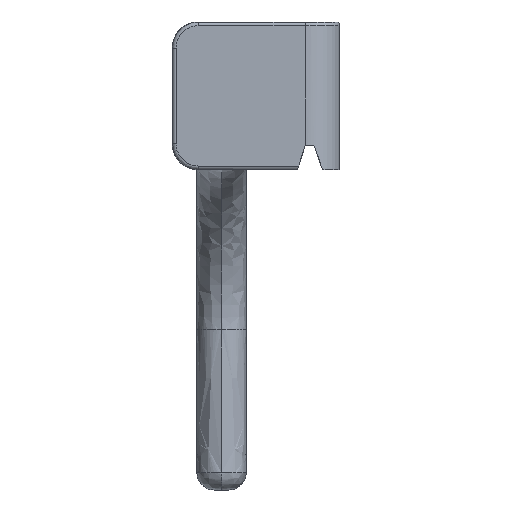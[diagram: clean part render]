
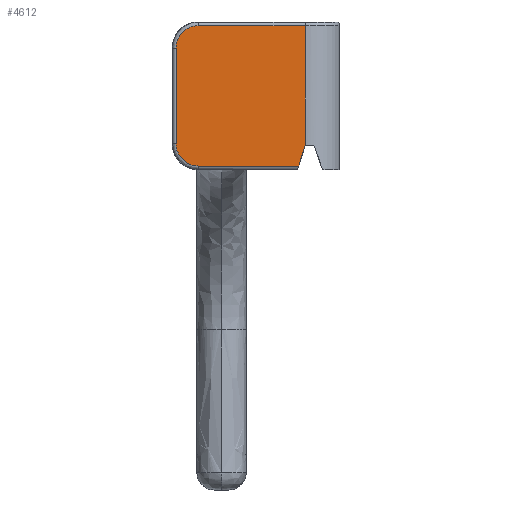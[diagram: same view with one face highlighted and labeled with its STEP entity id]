
A CAD part, front view. The second image highlights one B-rep face of the part: STEP entity #4612.
In plain terms, the highlighted planar face has unit normal (0, -1, 0).
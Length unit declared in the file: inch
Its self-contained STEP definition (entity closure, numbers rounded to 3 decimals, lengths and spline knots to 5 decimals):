
#20=PLANE('',#4950);
#330=FACE_OUTER_BOUND('',#638,.T.);
#638=EDGE_LOOP('',(#3064,#3065,#3066,#3067,#3068,#3069,#3070));
#939=B_SPLINE_CURVE_WITH_KNOTS('',3,(#5378,#5379,#5380,#5381,#5382,#5383),
 .UNSPECIFIED.,.F.,.F.,(4,1,1,4),(-0.71331,-0.40761,
-0.2038,0.),.UNSPECIFIED.);
#941=B_SPLINE_CURVE_WITH_KNOTS('',3,(#5429,#5430,#5431,#5432,#5433,#5434),
 .UNSPECIFIED.,.F.,.F.,(4,1,1,4),(-0.71331,-0.50951,
-0.3057,0.),.UNSPECIFIED.);
#1635=LINE('',#5343,#1679);
#1637=LINE('',#5394,#1681);
#1639=LINE('',#5445,#1683);
#1646=LINE('',#5490,#1690);
#1647=LINE('',#5497,#1691);
#1679=VECTOR('',#5064,0.3937);
#1681=VECTOR('',#5072,0.3937);
#1683=VECTOR('',#5080,0.3937);
#1690=VECTOR('',#5099,0.3937);
#1691=VECTOR('',#5108,0.3937);
#1769=VERTEX_POINT('',#5335);
#1771=VERTEX_POINT('',#5341);
#1773=VERTEX_POINT('',#5376);
#1775=VERTEX_POINT('',#5392);
#1777=VERTEX_POINT('',#5427);
#1779=VERTEX_POINT('',#5443);
#1788=VERTEX_POINT('',#5489);
#2237=EDGE_CURVE('',#1771,#1769,#1635,.T.);
#2240=EDGE_CURVE('',#1773,#1771,#939,.T.);
#2243=EDGE_CURVE('',#1775,#1773,#1637,.T.);
#2246=EDGE_CURVE('',#1777,#1775,#941,.T.);
#2249=EDGE_CURVE('',#1779,#1777,#1639,.T.);
#2261=EDGE_CURVE('',#1769,#1788,#1646,.T.);
#2265=EDGE_CURVE('',#1779,#1788,#1647,.T.);
#3064=ORIENTED_EDGE('',*,*,#2237,.F.);
#3065=ORIENTED_EDGE('',*,*,#2240,.F.);
#3066=ORIENTED_EDGE('',*,*,#2243,.F.);
#3067=ORIENTED_EDGE('',*,*,#2246,.F.);
#3068=ORIENTED_EDGE('',*,*,#2249,.F.);
#3069=ORIENTED_EDGE('',*,*,#2265,.T.);
#3070=ORIENTED_EDGE('',*,*,#2261,.F.);
#4612=ADVANCED_FACE('',(#330),#20,.T.);
#4950=AXIS2_PLACEMENT_3D('',#5496,#5106,#5107);
#5064=DIRECTION('',(1.,0.,0.));
#5072=DIRECTION('',(0.,0.,1.));
#5080=DIRECTION('',(-1.,0.,0.));
#5099=DIRECTION('',(0.,0.,-1.));
#5106=DIRECTION('center_axis',(0.,-1.,0.));
#5107=DIRECTION('ref_axis',(0.,0.,
-1.));
#5108=DIRECTION('',(0.3,0.,0.954));
#5335=CARTESIAN_POINT('',(0.6717,3.13929,-1.06923));
#5341=CARTESIAN_POINT('',(-0.18251,3.13929,-1.06923));
#5343=CARTESIAN_POINT('',(-0.19445,3.13929,-1.06923));
#5376=CARTESIAN_POINT('',(-0.3613,3.13929,-1.24802));
#5378=CARTESIAN_POINT('Ctrl Pts',(-0.3613,3.13929,-1.24802));
#5379=CARTESIAN_POINT('Ctrl Pts',(-0.3613,3.13929,-1.2079));
#5380=CARTESIAN_POINT('Ctrl Pts',(-0.33784,3.13929,-1.14128));
#5381=CARTESIAN_POINT('Ctrl Pts',(-0.26264,3.13929,-1.08147));
#5382=CARTESIAN_POINT('Ctrl Pts',(-0.20925,3.13929,-1.06923));
#5383=CARTESIAN_POINT('Ctrl Pts',(-0.18251,3.13929,-1.06923));
#5392=CARTESIAN_POINT('',(-0.3613,3.13929,-2.01154));
#5394=CARTESIAN_POINT('',(-0.3613,3.13929,-1.97427));
#5427=CARTESIAN_POINT('',(-0.18251,3.13929,-2.19033));
#5429=CARTESIAN_POINT('Ctrl Pts',(-0.18251,3.13929,-2.19033));
#5430=CARTESIAN_POINT('Ctrl Pts',(-0.20925,3.13929,-2.19033));
#5431=CARTESIAN_POINT('Ctrl Pts',(-0.26264,3.13929,-2.17809));
#5432=CARTESIAN_POINT('Ctrl Pts',(-0.33783,3.13929,-2.11828));
#5433=CARTESIAN_POINT('Ctrl Pts',(-0.3613,3.13929,-2.05166));
#5434=CARTESIAN_POINT('Ctrl Pts',(-0.3613,3.13929,-2.01154));
#5443=CARTESIAN_POINT('',(0.61918,3.13929,-2.19033));
#5445=CARTESIAN_POINT('',(-0.19445,3.13929,-2.19033));
#5489=CARTESIAN_POINT('',(0.6717,3.13929,-2.02348));
#5490=CARTESIAN_POINT('',(0.6717,3.13929,-1.3345));
#5496=CARTESIAN_POINT('Origin',(-0.19445,3.13929,-1.03923));
#5497=CARTESIAN_POINT('',(0.74261,3.13929,-1.79815));
